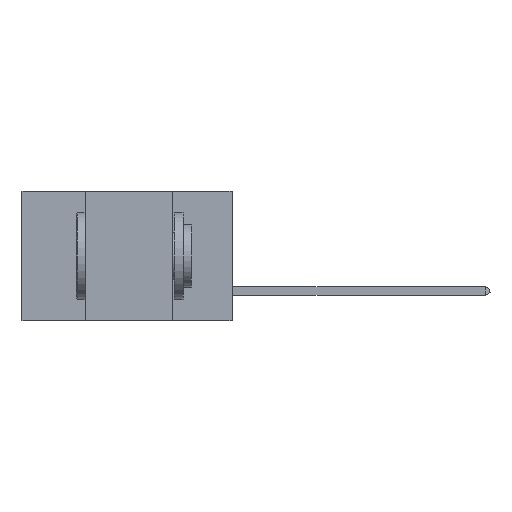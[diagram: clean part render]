
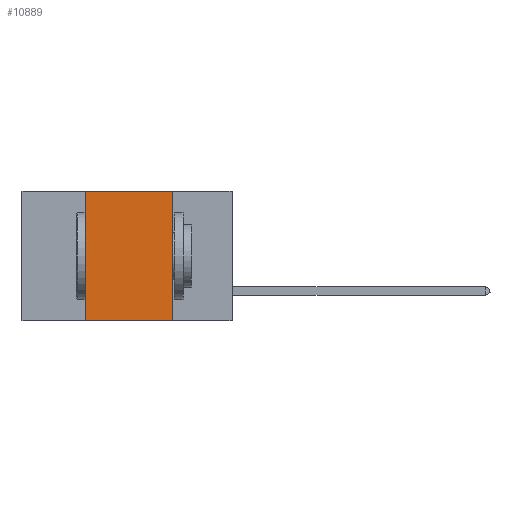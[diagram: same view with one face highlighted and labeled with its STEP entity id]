
A CAD part, left-side view. The second image highlights one B-rep face of the part: STEP entity #10889.
In plain terms, the highlighted planar face has unit normal (-1, 0, 0).
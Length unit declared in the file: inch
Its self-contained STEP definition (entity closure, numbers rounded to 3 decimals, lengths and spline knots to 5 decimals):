
#1238 = DIRECTION ( 'NONE',  ( 0., 0., 1. ) ) ;
#5366 = LINE ( 'NONE', #44984, #32963 ) ;
#6115 = VERTEX_POINT ( 'NONE', #38481 ) ;
#7135 = EDGE_CURVE ( 'NONE', #18682, #29904, #20056, .T. ) ;
#7272 = LINE ( 'NONE', #17414, #44444 ) ;
#8459 = VERTEX_POINT ( 'NONE', #16383 ) ;
#8696 = PLANE ( 'NONE',  #36771 ) ;
#9264 = EDGE_CURVE ( 'NONE', #6115, #8459, #7272, .T. ) ;
#10889 = ADVANCED_FACE ( 'NONE', ( #36947 ), #8696, .F. ) ;
#12489 = DIRECTION ( 'NONE',  ( 1., 0., 0. ) ) ;
#12714 = CARTESIAN_POINT ( 'NONE',  ( 0., 0.6, 0. ) ) ;
#16383 = CARTESIAN_POINT ( 'NONE',  ( 0., 0.17, -0.37 ) ) ;
#16863 = DIRECTION ( 'NONE',  ( 0., 0., -1. ) ) ;
#16876 = EDGE_CURVE ( 'NONE', #29904, #8459, #37520, .T. ) ;
#17133 = ORIENTED_EDGE ( 'NONE', *, *, #7135, .F. ) ;
#17414 = CARTESIAN_POINT ( 'NONE',  ( 0., 0.6, -0.37 ) ) ;
#17433 = ORIENTED_EDGE ( 'NONE', *, *, #30797, .F. ) ;
#18682 = VERTEX_POINT ( 'NONE', #23985 ) ;
#20056 = LINE ( 'NONE', #12714, #35288 ) ;
#23985 = CARTESIAN_POINT ( 'NONE',  ( 0., 0.42, 0. ) ) ;
#27027 = ORIENTED_EDGE ( 'NONE', *, *, #16876, .F. ) ;
#28105 = DIRECTION ( 'NONE',  ( 0., -1., 0. ) ) ;
#29904 = VERTEX_POINT ( 'NONE', #38999 ) ;
#30198 = VECTOR ( 'NONE', #16863, 39.37008 ) ;
#30797 = EDGE_CURVE ( 'NONE', #6115, #18682, #5366, .T. ) ;
#31486 = CARTESIAN_POINT ( 'NONE',  ( 0., 0.17, 0. ) ) ;
#32963 = VECTOR ( 'NONE', #1238, 39.37008 ) ;
#33899 = EDGE_LOOP ( 'NONE', ( #27027, #17133, #17433, #40538 ) ) ;
#34040 = CARTESIAN_POINT ( 'NONE',  ( 0., 0.6, 0. ) ) ;
#34122 = DIRECTION ( 'NONE',  ( 0., -1., 0. ) ) ;
#35288 = VECTOR ( 'NONE', #34122, 39.37008 ) ;
#36771 = AXIS2_PLACEMENT_3D ( 'NONE', #34040, #12489, #45199 ) ;
#36947 = FACE_OUTER_BOUND ( 'NONE', #33899, .T. ) ;
#37520 = LINE ( 'NONE', #31486, #30198 ) ;
#38481 = CARTESIAN_POINT ( 'NONE',  ( 0., 0.42, -0.37 ) ) ;
#38999 = CARTESIAN_POINT ( 'NONE',  ( 0., 0.17, 0. ) ) ;
#40538 = ORIENTED_EDGE ( 'NONE', *, *, #9264, .T. ) ;
#44444 = VECTOR ( 'NONE', #28105, 39.37008 ) ;
#44984 = CARTESIAN_POINT ( 'NONE',  ( 0., 0.42, 0. ) ) ;
#45199 = DIRECTION ( 'NONE',  ( 0., 0., -1. ) ) ;
